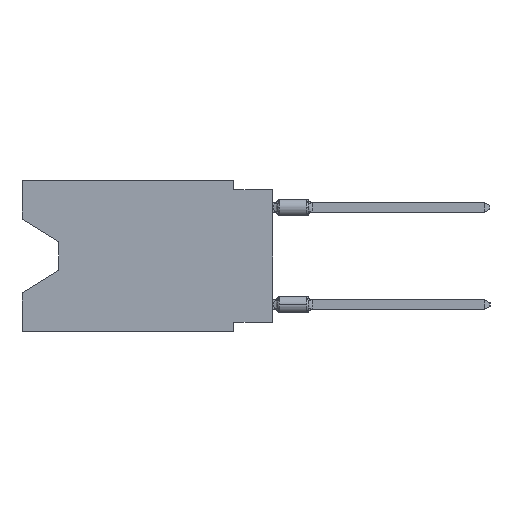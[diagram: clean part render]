
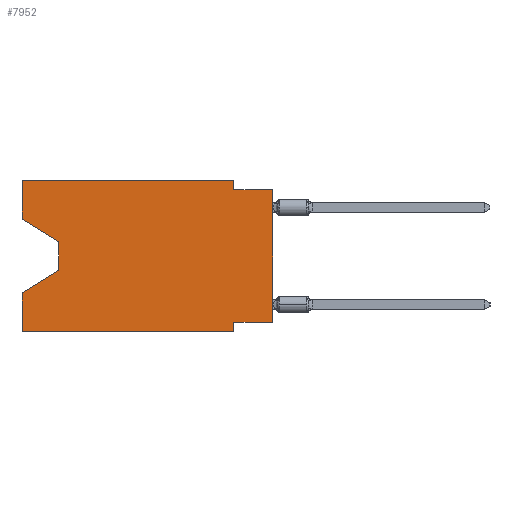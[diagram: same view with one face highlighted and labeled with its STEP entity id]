
A CAD part, left-side view. The second image highlights one B-rep face of the part: STEP entity #7952.
In plain terms, the highlighted planar face has unit normal (-1, 0, 0).
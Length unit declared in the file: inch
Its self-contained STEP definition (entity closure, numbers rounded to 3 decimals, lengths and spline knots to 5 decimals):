
#96 = CARTESIAN_POINT ( 'NONE',  ( 0., 0.645, 0. ) ) ;
#135 = VERTEX_POINT ( 'NONE', #20917 ) ;
#431 = VERTEX_POINT ( 'NONE', #4336 ) ;
#1151 = CARTESIAN_POINT ( 'NONE',  ( 0., 0.645, -0.39 ) ) ;
#1235 = CARTESIAN_POINT ( 'NONE',  ( 0., 0.645, 0. ) ) ;
#1489 = EDGE_CURVE ( 'NONE', #16074, #431, #29089, .T. ) ;
#1560 = ORIENTED_EDGE ( 'NONE', *, *, #12126, .F. ) ;
#2456 = CARTESIAN_POINT ( 'NONE',  ( 0., 0.1, -0.39 ) ) ;
#3898 = EDGE_CURVE ( 'NONE', #14419, #5379, #28376, .T. ) ;
#4193 = LINE ( 'NONE', #1151, #25289 ) ;
#4207 = ORIENTED_EDGE ( 'NONE', *, *, #18531, .F. ) ;
#4336 = CARTESIAN_POINT ( 'NONE',  ( 0., 0.645, -0.28975 ) ) ;
#4602 = ORIENTED_EDGE ( 'NONE', *, *, #15976, .T. ) ;
#5379 = VERTEX_POINT ( 'NONE', #8622 ) ;
#5708 = VECTOR ( 'NONE', #18131, 39.37008 ) ;
#6256 = CARTESIAN_POINT ( 'NONE',  ( 0., 0.645, -0.39 ) ) ;
#6642 = ORIENTED_EDGE ( 'NONE', *, *, #24122, .F. ) ;
#6793 = DIRECTION ( 'NONE',  ( 0., 0., 1. ) ) ;
#6823 = DIRECTION ( 'NONE',  ( 0., 1., 0. ) ) ;
#7006 = CARTESIAN_POINT ( 'NONE',  ( 0., 0., -0.365 ) ) ;
#7793 = VERTEX_POINT ( 'NONE', #27505 ) ;
#7928 = EDGE_CURVE ( 'NONE', #16074, #27677, #4193, .T. ) ;
#7952 = ADVANCED_FACE ( 'NONE', ( #12613 ), #23580, .F. ) ;
#7988 = DIRECTION ( 'NONE',  ( 0., 0., 1. ) ) ;
#8622 = CARTESIAN_POINT ( 'NONE',  ( 0., 0.55, -0.158 ) ) ;
#8774 = EDGE_CURVE ( 'NONE', #23420, #29322, #29077, .T. ) ;
#8837 = DIRECTION ( 'NONE',  ( 0., -0.855, -0.519 ) ) ;
#8884 = VECTOR ( 'NONE', #6823, 39.37008 ) ;
#9867 = LINE ( 'NONE', #12544, #17852 ) ;
#9931 = DIRECTION ( 'NONE',  ( 1., 0., 0. ) ) ;
#10669 = CARTESIAN_POINT ( 'NONE',  ( 0., 0.1, -0.025 ) ) ;
#11224 = ORIENTED_EDGE ( 'NONE', *, *, #1489, .F. ) ;
#11512 = VECTOR ( 'NONE', #7988, 39.37008 ) ;
#12083 = DIRECTION ( 'NONE',  ( 0., -1., 0. ) ) ;
#12126 = EDGE_CURVE ( 'NONE', #14419, #7793, #32366, .T. ) ;
#12337 = CARTESIAN_POINT ( 'NONE',  ( 0., 0.1, 0. ) ) ;
#12383 = LINE ( 'NONE', #23699, #22742 ) ;
#12544 = CARTESIAN_POINT ( 'NONE',  ( 0., 0.1, 0. ) ) ;
#12613 = FACE_OUTER_BOUND ( 'NONE', #17614, .T. ) ;
#12935 = CARTESIAN_POINT ( 'NONE',  ( 0., 0.645, 0. ) ) ;
#12944 = EDGE_CURVE ( 'NONE', #135, #27677, #24034, .T. ) ;
#13963 = ORIENTED_EDGE ( 'NONE', *, *, #3898, .T. ) ;
#14334 = VERTEX_POINT ( 'NONE', #12337 ) ;
#14419 = VERTEX_POINT ( 'NONE', #15568 ) ;
#14872 = CARTESIAN_POINT ( 'NONE',  ( 0., 0., 0. ) ) ;
#14889 = CARTESIAN_POINT ( 'NONE',  ( 0., 0.55, -0.158 ) ) ;
#14999 = ORIENTED_EDGE ( 'NONE', *, *, #12944, .F. ) ;
#15568 = CARTESIAN_POINT ( 'NONE',  ( 0., 0.645, -0.10025 ) ) ;
#15588 = ORIENTED_EDGE ( 'NONE', *, *, #19925, .T. ) ;
#15976 = EDGE_CURVE ( 'NONE', #20891, #29322, #22956, .T. ) ;
#16074 = VERTEX_POINT ( 'NONE', #6256 ) ;
#16721 = VECTOR ( 'NONE', #30096, 39.37008 ) ;
#17614 = EDGE_LOOP ( 'NONE', ( #13963, #22052, #15588, #11224, #31610, #14999, #4207, #4602, #21927, #26554, #6642, #1560 ) ) ;
#17852 = VECTOR ( 'NONE', #23344, 39.37008 ) ;
#17933 = LINE ( 'NONE', #7006, #8884 ) ;
#17947 = CARTESIAN_POINT ( 'NONE',  ( 0., 0., -0.025 ) ) ;
#18090 = DIRECTION ( 'NONE',  ( 0., -1., 0. ) ) ;
#18131 = DIRECTION ( 'NONE',  ( 0., -1., 0. ) ) ;
#18462 = DIRECTION ( 'NONE',  ( 0., 0.855, -0.519 ) ) ;
#18531 = EDGE_CURVE ( 'NONE', #20891, #135, #17933, .T. ) ;
#18924 = CARTESIAN_POINT ( 'NONE',  ( 0., 0., -0.025 ) ) ;
#19163 = CARTESIAN_POINT ( 'NONE',  ( 0., 0.1, -0.39 ) ) ;
#19925 = EDGE_CURVE ( 'NONE', #31050, #431, #12383, .T. ) ;
#20874 = DIRECTION ( 'NONE',  ( 0., 0., -1. ) ) ;
#20891 = VERTEX_POINT ( 'NONE', #31777 ) ;
#20917 = CARTESIAN_POINT ( 'NONE',  ( 0., 0.1, -0.365 ) ) ;
#21208 = VECTOR ( 'NONE', #23719, 39.37008 ) ;
#21472 = VECTOR ( 'NONE', #6793, 39.37008 ) ;
#21927 = ORIENTED_EDGE ( 'NONE', *, *, #8774, .F. ) ;
#22052 = ORIENTED_EDGE ( 'NONE', *, *, #30382, .T. ) ;
#22742 = VECTOR ( 'NONE', #18462, 39.37008 ) ;
#22956 = LINE ( 'NONE', #14872, #21472 ) ;
#23344 = DIRECTION ( 'NONE',  ( 0., 0., -1. ) ) ;
#23380 = CARTESIAN_POINT ( 'NONE',  ( 0., 0.645, -0.10025 ) ) ;
#23420 = VERTEX_POINT ( 'NONE', #10669 ) ;
#23580 = PLANE ( 'NONE',  #26996 ) ;
#23699 = CARTESIAN_POINT ( 'NONE',  ( 0., 0.55, -0.232 ) ) ;
#23719 = DIRECTION ( 'NONE',  ( 0., 0., 1. ) ) ;
#24034 = LINE ( 'NONE', #19163, #16721 ) ;
#24122 = EDGE_CURVE ( 'NONE', #7793, #14334, #31537, .T. ) ;
#24140 = VECTOR ( 'NONE', #18090, 39.37008 ) ;
#24570 = EDGE_CURVE ( 'NONE', #14334, #23420, #9867, .T. ) ;
#25289 = VECTOR ( 'NONE', #12083, 39.37008 ) ;
#25655 = DIRECTION ( 'NONE',  ( 0., 0., -1. ) ) ;
#26554 = ORIENTED_EDGE ( 'NONE', *, *, #24570, .F. ) ;
#26996 = AXIS2_PLACEMENT_3D ( 'NONE', #34502, #9931, #20874 ) ;
#27505 = CARTESIAN_POINT ( 'NONE',  ( 0., 0.645, 0. ) ) ;
#27677 = VERTEX_POINT ( 'NONE', #2456 ) ;
#28376 = LINE ( 'NONE', #23380, #30435 ) ;
#29077 = LINE ( 'NONE', #17947, #5708 ) ;
#29089 = LINE ( 'NONE', #12935, #21208 ) ;
#29322 = VERTEX_POINT ( 'NONE', #18924 ) ;
#29472 = VECTOR ( 'NONE', #25655, 39.37008 ) ;
#30096 = DIRECTION ( 'NONE',  ( 0., 0., -1. ) ) ;
#30382 = EDGE_CURVE ( 'NONE', #5379, #31050, #31547, .T. ) ;
#30435 = VECTOR ( 'NONE', #8837, 39.37008 ) ;
#30574 = CARTESIAN_POINT ( 'NONE',  ( 0., 0.55, -0.232 ) ) ;
#31050 = VERTEX_POINT ( 'NONE', #30574 ) ;
#31537 = LINE ( 'NONE', #1235, #24140 ) ;
#31547 = LINE ( 'NONE', #14889, #29472 ) ;
#31610 = ORIENTED_EDGE ( 'NONE', *, *, #7928, .T. ) ;
#31777 = CARTESIAN_POINT ( 'NONE',  ( 0., 0., -0.365 ) ) ;
#32366 = LINE ( 'NONE', #96, #11512 ) ;
#34502 = CARTESIAN_POINT ( 'NONE',  ( 0., 0.645, 0. ) ) ;
